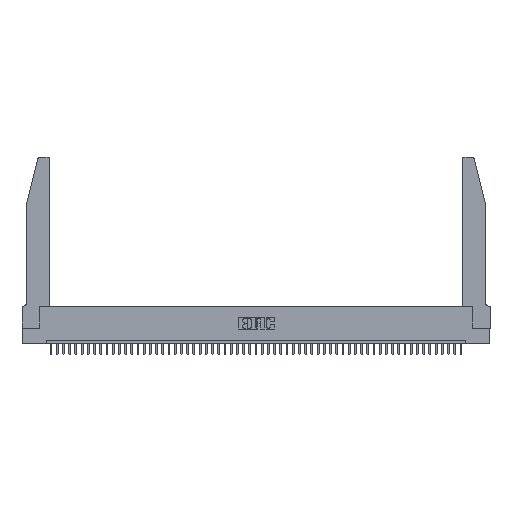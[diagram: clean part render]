
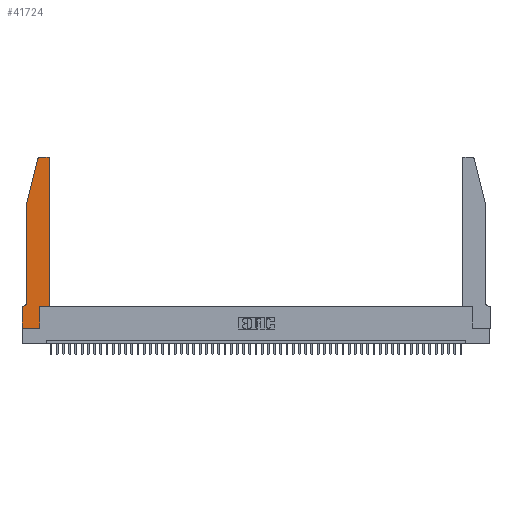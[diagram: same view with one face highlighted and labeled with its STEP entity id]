
A CAD part, top view. The second image highlights one B-rep face of the part: STEP entity #41724.
In plain terms, the highlighted planar face has unit normal (0, 0, 1).
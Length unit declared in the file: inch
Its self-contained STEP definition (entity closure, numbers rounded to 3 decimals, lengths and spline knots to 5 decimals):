
#552 = LINE ( 'NONE', #49941, #45655 ) ;
#557 = CARTESIAN_POINT ( 'NONE',  ( 0.0755, 2., 0.37 ) ) ;
#1644 = CARTESIAN_POINT ( 'NONE',  ( 0., 0.35, 0.37 ) ) ;
#1693 = CARTESIAN_POINT ( 'NONE',  ( 0.2865, 0.35, 0.37 ) ) ;
#2271 = CARTESIAN_POINT ( 'NONE',  ( 0.4205, 2.72, 0.37 ) ) ;
#2784 = FACE_OUTER_BOUND ( 'NONE', #47410, .T. ) ;
#4338 = CARTESIAN_POINT ( 'NONE',  ( 0.2865, 0.35, 0.37 ) ) ;
#4614 = CIRCLE ( 'NONE', #44169, 0.07 ) ;
#4809 = DIRECTION ( 'NONE',  ( 1., 0., 0. ) ) ;
#4883 = CARTESIAN_POINT ( 'NONE',  ( 0.4205, 2.75, 0.37 ) ) ;
#5109 = DIRECTION ( 'NONE',  ( 0., 0., 1. ) ) ;
#5362 = VECTOR ( 'NONE', #34049, 39.37008 ) ;
#5997 = VERTEX_POINT ( 'NONE', #9059 ) ;
#6088 = DIRECTION ( 'NONE',  ( 0., 0., 1. ) ) ;
#6496 = VERTEX_POINT ( 'NONE', #7644 ) ;
#6665 = DIRECTION ( 'NONE',  ( -0.239, -0.971, 0. ) ) ;
#6702 = ORIENTED_EDGE ( 'NONE', *, *, #31625, .T. ) ;
#7644 = CARTESIAN_POINT ( 'NONE',  ( 0.4505, 2.72, 0.37 ) ) ;
#9059 = CARTESIAN_POINT ( 'NONE',  ( 0.4505, 0.35, 0.37 ) ) ;
#9338 = CARTESIAN_POINT ( 'NONE',  ( 0.0755, 2., 0.37 ) ) ;
#9586 = CARTESIAN_POINT ( 'NONE',  ( 0.0055, 0.35, 0.37 ) ) ;
#9799 = VERTEX_POINT ( 'NONE', #1693 ) ;
#10500 = AXIS2_PLACEMENT_3D ( 'NONE', #51434, #31232, #26834 ) ;
#10527 = CARTESIAN_POINT ( 'NONE',  ( 0.2605, 2.75, 0.37 ) ) ;
#11130 = VECTOR ( 'NONE', #6665, 39.37008 ) ;
#11403 = ORIENTED_EDGE ( 'NONE', *, *, #51018, .T. ) ;
#11781 = ORIENTED_EDGE ( 'NONE', *, *, #12588, .T. ) ;
#11975 = CIRCLE ( 'NONE', #10500, 0.03 ) ;
#12283 = EDGE_CURVE ( 'NONE', #43551, #30245, #43088, .T. ) ;
#12588 = EDGE_CURVE ( 'NONE', #24158, #22667, #29180, .T. ) ;
#12879 = CARTESIAN_POINT ( 'NONE',  ( 0.0755, 0.42, 0.37 ) ) ;
#12938 = DIRECTION ( 'NONE',  ( 0., 1., 0. ) ) ;
#13551 = VECTOR ( 'NONE', #32597, 39.37008 ) ;
#13563 = DIRECTION ( 'NONE',  ( 1., 0., 0. ) ) ;
#14135 = ORIENTED_EDGE ( 'NONE', *, *, #30301, .T. ) ;
#14239 = ORIENTED_EDGE ( 'NONE', *, *, #12283, .T. ) ;
#15993 = EDGE_CURVE ( 'NONE', #17157, #43551, #11975, .T. ) ;
#16612 = ORIENTED_EDGE ( 'NONE', *, *, #15993, .T. ) ;
#17157 = VERTEX_POINT ( 'NONE', #26160 ) ;
#17827 = DIRECTION ( 'NONE',  ( -1., 0., 0. ) ) ;
#17992 = LINE ( 'NONE', #557, #13551 ) ;
#18628 = ORIENTED_EDGE ( 'NONE', *, *, #49102, .T. ) ;
#19755 = EDGE_CURVE ( 'NONE', #29446, #9799, #44994, .T. ) ;
#21680 = CARTESIAN_POINT ( 'NONE',  ( 0.0755, 0.35, 0.37 ) ) ;
#21819 = VECTOR ( 'NONE', #27027, 39.37008 ) ;
#22067 = DIRECTION ( 'NONE',  ( 1., 0., 0. ) ) ;
#22221 = DIRECTION ( 'NONE',  ( 0., 0., -1. ) ) ;
#22455 = VECTOR ( 'NONE', #12938, 39.37008 ) ;
#22667 = VERTEX_POINT ( 'NONE', #51647 ) ;
#23196 = EDGE_CURVE ( 'NONE', #5997, #6496, #25162, .T. ) ;
#24158 = VERTEX_POINT ( 'NONE', #31274 ) ;
#24909 = VECTOR ( 'NONE', #49746, 39.37008 ) ;
#24945 = AXIS2_PLACEMENT_3D ( 'NONE', #1644, #5109, #13563 ) ;
#25162 = LINE ( 'NONE', #27437, #34629 ) ;
#25346 = EDGE_CURVE ( 'NONE', #30245, #25624, #17992, .T. ) ;
#25441 = PLANE ( 'NONE',  #24945 ) ;
#25624 = VERTEX_POINT ( 'NONE', #12879 ) ;
#26160 = CARTESIAN_POINT ( 'NONE',  ( 0.284, 2.75, 0.37 ) ) ;
#26834 = DIRECTION ( 'NONE',  ( 1., 0., 0. ) ) ;
#27027 = DIRECTION ( 'NONE',  ( 1., 0., 0. ) ) ;
#27069 = ORIENTED_EDGE ( 'NONE', *, *, #38542, .T. ) ;
#27437 = CARTESIAN_POINT ( 'NONE',  ( 0.4505, 0.35, 0.37 ) ) ;
#28252 = CARTESIAN_POINT ( 'NONE',  ( 0.2865, 0., 0.37 ) ) ;
#28675 = LINE ( 'NONE', #50392, #21819 ) ;
#29180 = LINE ( 'NONE', #45971, #5362 ) ;
#29446 = VERTEX_POINT ( 'NONE', #28252 ) ;
#30245 = VERTEX_POINT ( 'NONE', #42837 ) ;
#30283 = DIRECTION ( 'NONE',  ( -1., 0., 0. ) ) ;
#30301 = EDGE_CURVE ( 'NONE', #6496, #35425, #33744, .T. ) ;
#31232 = DIRECTION ( 'NONE',  ( 0., 0., 1. ) ) ;
#31274 = CARTESIAN_POINT ( 'NONE',  ( 0., 0.35, 0.37 ) ) ;
#31625 = EDGE_CURVE ( 'NONE', #35425, #17157, #47718, .T. ) ;
#32597 = DIRECTION ( 'NONE',  ( 0., -1., 0. ) ) ;
#33304 = ORIENTED_EDGE ( 'NONE', *, *, #25346, .T. ) ;
#33744 = CIRCLE ( 'NONE', #42935, 0.03 ) ;
#34049 = DIRECTION ( 'NONE',  ( 0., -1., 0. ) ) ;
#34629 = VECTOR ( 'NONE', #43936, 39.37008 ) ;
#35420 = ORIENTED_EDGE ( 'NONE', *, *, #23196, .T. ) ;
#35425 = VERTEX_POINT ( 'NONE', #4883 ) ;
#38194 = LINE ( 'NONE', #21680, #24909 ) ;
#38542 = EDGE_CURVE ( 'NONE', #9799, #5997, #28675, .T. ) ;
#41724 = ADVANCED_FACE ( 'NONE', ( #2784 ), #25441, .T. ) ;
#41810 = CARTESIAN_POINT ( 'NONE',  ( 0.0055, 0.42, 0.37 ) ) ;
#42837 = CARTESIAN_POINT ( 'NONE',  ( 0.0755, 2., 0.37 ) ) ;
#42935 = AXIS2_PLACEMENT_3D ( 'NONE', #2271, #6088, #4809 ) ;
#43088 = LINE ( 'NONE', #9338, #11130 ) ;
#43551 = VERTEX_POINT ( 'NONE', #45924 ) ;
#43936 = DIRECTION ( 'NONE',  ( 0., 1., 0. ) ) ;
#44126 = EDGE_CURVE ( 'NONE', #25624, #46511, #4614, .T. ) ;
#44169 = AXIS2_PLACEMENT_3D ( 'NONE', #41810, #22221, #17827 ) ;
#44994 = LINE ( 'NONE', #4338, #22455 ) ;
#45655 = VECTOR ( 'NONE', #22067, 39.37008 ) ;
#45924 = CARTESIAN_POINT ( 'NONE',  ( 0.25487, 2.72718, 0.37 ) ) ;
#45971 = CARTESIAN_POINT ( 'NONE',  ( 0., 0., 0.37 ) ) ;
#46466 = VECTOR ( 'NONE', #30283, 39.37008 ) ;
#46511 = VERTEX_POINT ( 'NONE', #9586 ) ;
#47410 = EDGE_LOOP ( 'NONE', ( #6702, #16612, #14239, #33304, #49874, #11403, #11781, #18628, #48105, #27069, #35420, #14135 ) ) ;
#47718 = LINE ( 'NONE', #10527, #46466 ) ;
#48105 = ORIENTED_EDGE ( 'NONE', *, *, #19755, .T. ) ;
#49102 = EDGE_CURVE ( 'NONE', #22667, #29446, #552, .T. ) ;
#49746 = DIRECTION ( 'NONE',  ( -1., 0., 0. ) ) ;
#49874 = ORIENTED_EDGE ( 'NONE', *, *, #44126, .T. ) ;
#49941 = CARTESIAN_POINT ( 'NONE',  ( 0., 0., 0.37 ) ) ;
#50392 = CARTESIAN_POINT ( 'NONE',  ( 0.4505, 0.35, 0.37 ) ) ;
#51018 = EDGE_CURVE ( 'NONE', #46511, #24158, #38194, .T. ) ;
#51434 = CARTESIAN_POINT ( 'NONE',  ( 0.284, 2.72, 0.37 ) ) ;
#51647 = CARTESIAN_POINT ( 'NONE',  ( 0., 0., 0.37 ) ) ;
